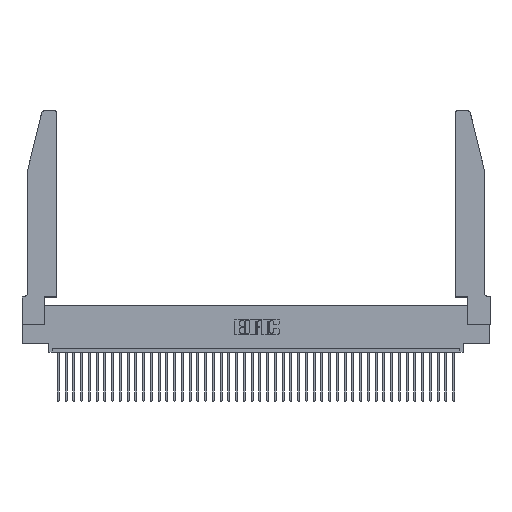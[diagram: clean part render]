
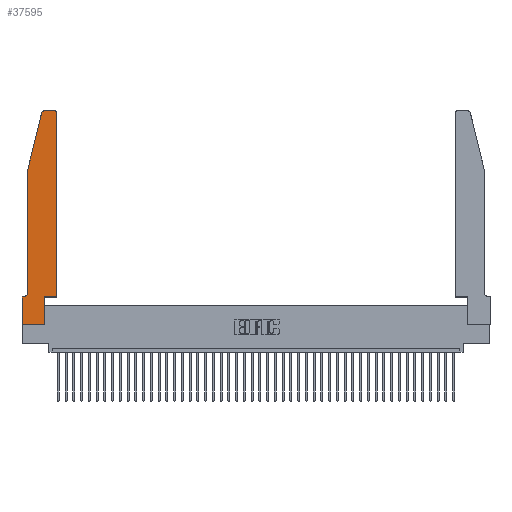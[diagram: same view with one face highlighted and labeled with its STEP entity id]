
A CAD part, top view. The second image highlights one B-rep face of the part: STEP entity #37595.
In plain terms, the highlighted planar face has unit normal (0, 0, 1).
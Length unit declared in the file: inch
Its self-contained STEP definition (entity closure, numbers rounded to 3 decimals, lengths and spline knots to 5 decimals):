
#277 = EDGE_CURVE ( 'NONE', #40830, #7163, #21932, .T. ) ;
#450 = DIRECTION ( 'NONE',  ( 0., -1., 0. ) ) ;
#536 = AXIS2_PLACEMENT_3D ( 'NONE', #16765, #16617, #23593 ) ;
#1195 = VECTOR ( 'NONE', #23611, 39.37008 ) ;
#1420 = DIRECTION ( 'NONE',  ( 0., 0., 1. ) ) ;
#1421 = CIRCLE ( 'NONE', #24104, 0.03 ) ;
#1528 = VECTOR ( 'NONE', #5284, 39.37008 ) ;
#1737 = CARTESIAN_POINT ( 'NONE',  ( 0.0055, 0.35, 0.37 ) ) ;
#1803 = DIRECTION ( 'NONE',  ( 0., 1., 0. ) ) ;
#1921 = CARTESIAN_POINT ( 'NONE',  ( 0.4505, 0.35, 0.37 ) ) ;
#2567 = VERTEX_POINT ( 'NONE', #10503 ) ;
#3373 = LINE ( 'NONE', #39535, #5455 ) ;
#4982 = ORIENTED_EDGE ( 'NONE', *, *, #31896, .T. ) ;
#5023 = VERTEX_POINT ( 'NONE', #1737 ) ;
#5186 = ORIENTED_EDGE ( 'NONE', *, *, #26673, .T. ) ;
#5284 = DIRECTION ( 'NONE',  ( 1., 0., 0. ) ) ;
#5455 = VECTOR ( 'NONE', #450, 39.37008 ) ;
#5745 = VERTEX_POINT ( 'NONE', #25918 ) ;
#5803 = EDGE_CURVE ( 'NONE', #5023, #11885, #7084, .T. ) ;
#6230 = CARTESIAN_POINT ( 'NONE',  ( 0.4205, 2.75, 0.37 ) ) ;
#6585 = VECTOR ( 'NONE', #26389, 39.37008 ) ;
#6752 = VERTEX_POINT ( 'NONE', #1921 ) ;
#7084 = LINE ( 'NONE', #29319, #11212 ) ;
#7163 = VERTEX_POINT ( 'NONE', #25752 ) ;
#7357 = DIRECTION ( 'NONE',  ( 0., 0., 1. ) ) ;
#7606 = CARTESIAN_POINT ( 'NONE',  ( 0.4505, 0.35, 0.37 ) ) ;
#9403 = EDGE_CURVE ( 'NONE', #33186, #11996, #1421, .T. ) ;
#9926 = LINE ( 'NONE', #39870, #1195 ) ;
#10177 = ORIENTED_EDGE ( 'NONE', *, *, #42155, .T. ) ;
#10503 = CARTESIAN_POINT ( 'NONE',  ( 0., 0., 0.37 ) ) ;
#11210 = CARTESIAN_POINT ( 'NONE',  ( 0.4505, 2.72, 0.37 ) ) ;
#11212 = VECTOR ( 'NONE', #16201, 39.37008 ) ;
#11885 = VERTEX_POINT ( 'NONE', #38442 ) ;
#11996 = VERTEX_POINT ( 'NONE', #6230 ) ;
#12301 = ORIENTED_EDGE ( 'NONE', *, *, #24446, .T. ) ;
#12445 = CARTESIAN_POINT ( 'NONE',  ( 0.0755, 0.42, 0.37 ) ) ;
#14690 = LINE ( 'NONE', #31631, #40524 ) ;
#14922 = FACE_OUTER_BOUND ( 'NONE', #30557, .T. ) ;
#14957 = DIRECTION ( 'NONE',  ( 1., 0., 0. ) ) ;
#16070 = LINE ( 'NONE', #25490, #23334 ) ;
#16130 = VERTEX_POINT ( 'NONE', #21897 ) ;
#16201 = DIRECTION ( 'NONE',  ( -1., 0., 0. ) ) ;
#16413 = AXIS2_PLACEMENT_3D ( 'NONE', #23859, #7357, #30424 ) ;
#16617 = DIRECTION ( 'NONE',  ( 0., 0., -1. ) ) ;
#16765 = CARTESIAN_POINT ( 'NONE',  ( 0.0055, 0.42, 0.37 ) ) ;
#17606 = ORIENTED_EDGE ( 'NONE', *, *, #29508, .T. ) ;
#17853 = CARTESIAN_POINT ( 'NONE',  ( 0.4205, 2.72, 0.37 ) ) ;
#17954 = ORIENTED_EDGE ( 'NONE', *, *, #39475, .T. ) ;
#18091 = EDGE_CURVE ( 'NONE', #7163, #6752, #18704, .T. ) ;
#18704 = LINE ( 'NONE', #7606, #24396 ) ;
#19626 = VERTEX_POINT ( 'NONE', #36937 ) ;
#19827 = PLANE ( 'NONE',  #22035 ) ;
#20003 = ORIENTED_EDGE ( 'NONE', *, *, #5803, .T. ) ;
#20592 = LINE ( 'NONE', #22306, #1528 ) ;
#21835 = CARTESIAN_POINT ( 'NONE',  ( 0.2865, 0., 0.37 ) ) ;
#21897 = CARTESIAN_POINT ( 'NONE',  ( 0.25487, 2.72718, 0.37 ) ) ;
#21932 = LINE ( 'NONE', #25497, #27052 ) ;
#22035 = AXIS2_PLACEMENT_3D ( 'NONE', #33332, #23188, #26888 ) ;
#22306 = CARTESIAN_POINT ( 'NONE',  ( 0., 0., 0.37 ) ) ;
#23188 = DIRECTION ( 'NONE',  ( 0., 0., 1. ) ) ;
#23334 = VECTOR ( 'NONE', #1803, 39.37008 ) ;
#23593 = DIRECTION ( 'NONE',  ( -1., 0., 0. ) ) ;
#23611 = DIRECTION ( 'NONE',  ( 0., -1., 0. ) ) ;
#23859 = CARTESIAN_POINT ( 'NONE',  ( 0.284, 2.72, 0.37 ) ) ;
#24104 = AXIS2_PLACEMENT_3D ( 'NONE', #17853, #1420, #14957 ) ;
#24396 = VECTOR ( 'NONE', #30679, 39.37008 ) ;
#24446 = EDGE_CURVE ( 'NONE', #11996, #19626, #14690, .T. ) ;
#25490 = CARTESIAN_POINT ( 'NONE',  ( 0.4505, 0.35, 0.37 ) ) ;
#25497 = CARTESIAN_POINT ( 'NONE',  ( 0.2865, 0.35, 0.37 ) ) ;
#25680 = ORIENTED_EDGE ( 'NONE', *, *, #35999, .T. ) ;
#25752 = CARTESIAN_POINT ( 'NONE',  ( 0.2865, 0.35, 0.37 ) ) ;
#25833 = ORIENTED_EDGE ( 'NONE', *, *, #40970, .T. ) ;
#25918 = CARTESIAN_POINT ( 'NONE',  ( 0.0755, 2., 0.37 ) ) ;
#26389 = DIRECTION ( 'NONE',  ( -0.239, -0.971, 0. ) ) ;
#26673 = EDGE_CURVE ( 'NONE', #5745, #34447, #9926, .T. ) ;
#26888 = DIRECTION ( 'NONE',  ( 1., 0., 0. ) ) ;
#27052 = VECTOR ( 'NONE', #38271, 39.37008 ) ;
#29319 = CARTESIAN_POINT ( 'NONE',  ( 0.0755, 0.35, 0.37 ) ) ;
#29508 = EDGE_CURVE ( 'NONE', #34447, #5023, #36994, .T. ) ;
#29685 = CARTESIAN_POINT ( 'NONE',  ( 0.0755, 2., 0.37 ) ) ;
#30424 = DIRECTION ( 'NONE',  ( 1., 0., 0. ) ) ;
#30557 = EDGE_LOOP ( 'NONE', ( #12301, #10177, #25833, #5186, #17606, #20003, #4982, #17954, #42662, #38232, #25680, #40452 ) ) ;
#30679 = DIRECTION ( 'NONE',  ( 1., 0., 0. ) ) ;
#31631 = CARTESIAN_POINT ( 'NONE',  ( 0.2605, 2.75, 0.37 ) ) ;
#31873 = LINE ( 'NONE', #29685, #6585 ) ;
#31896 = EDGE_CURVE ( 'NONE', #11885, #2567, #3373, .T. ) ;
#33186 = VERTEX_POINT ( 'NONE', #11210 ) ;
#33332 = CARTESIAN_POINT ( 'NONE',  ( 0., 0.35, 0.37 ) ) ;
#34447 = VERTEX_POINT ( 'NONE', #12445 ) ;
#35999 = EDGE_CURVE ( 'NONE', #6752, #33186, #16070, .T. ) ;
#36937 = CARTESIAN_POINT ( 'NONE',  ( 0.284, 2.75, 0.37 ) ) ;
#36994 = CIRCLE ( 'NONE', #536, 0.07 ) ;
#37436 = CIRCLE ( 'NONE', #16413, 0.03 ) ;
#37595 = ADVANCED_FACE ( 'NONE', ( #14922 ), #19827, .T. ) ;
#38232 = ORIENTED_EDGE ( 'NONE', *, *, #18091, .T. ) ;
#38271 = DIRECTION ( 'NONE',  ( 0., 1., 0. ) ) ;
#38442 = CARTESIAN_POINT ( 'NONE',  ( 0., 0.35, 0.37 ) ) ;
#39475 = EDGE_CURVE ( 'NONE', #2567, #40830, #20592, .T. ) ;
#39535 = CARTESIAN_POINT ( 'NONE',  ( 0., 0., 0.37 ) ) ;
#39870 = CARTESIAN_POINT ( 'NONE',  ( 0.0755, 2., 0.37 ) ) ;
#40452 = ORIENTED_EDGE ( 'NONE', *, *, #9403, .T. ) ;
#40524 = VECTOR ( 'NONE', #41443, 39.37008 ) ;
#40830 = VERTEX_POINT ( 'NONE', #21835 ) ;
#40970 = EDGE_CURVE ( 'NONE', #16130, #5745, #31873, .T. ) ;
#41443 = DIRECTION ( 'NONE',  ( -1., 0., 0. ) ) ;
#42155 = EDGE_CURVE ( 'NONE', #19626, #16130, #37436, .T. ) ;
#42662 = ORIENTED_EDGE ( 'NONE', *, *, #277, .T. ) ;
